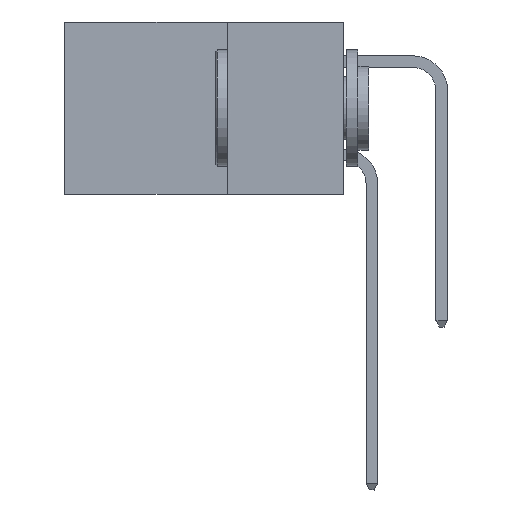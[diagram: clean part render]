
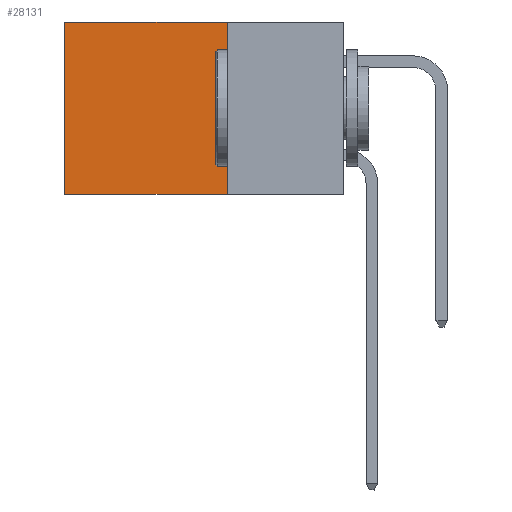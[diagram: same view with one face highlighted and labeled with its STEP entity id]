
A CAD part, left-side view. The second image highlights one B-rep face of the part: STEP entity #28131.
In plain terms, the highlighted planar face has unit normal (-1, 0, 0).
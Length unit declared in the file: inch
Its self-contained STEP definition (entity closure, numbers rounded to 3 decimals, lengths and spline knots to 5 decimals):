
#2382 = VECTOR ( 'NONE', #5284, 39.37008 ) ;
#3113 = CARTESIAN_POINT ( 'NONE',  ( 0.298, 0.6, 0. ) ) ;
#5284 = DIRECTION ( 'NONE',  ( 0., 0., -1. ) ) ;
#5970 = DIRECTION ( 'NONE',  ( 1., 0., 0. ) ) ;
#7076 = LINE ( 'NONE', #7590, #25088 ) ;
#7232 = CARTESIAN_POINT ( 'NONE',  ( 0.298, 0.25, -0.37 ) ) ;
#7590 = CARTESIAN_POINT ( 'NONE',  ( 0.298, 0.6, 0. ) ) ;
#7758 = VERTEX_POINT ( 'NONE', #3113 ) ;
#7760 = CARTESIAN_POINT ( 'NONE',  ( 0.298, 0.25, 0. ) ) ;
#7914 = ORIENTED_EDGE ( 'NONE', *, *, #15413, .T. ) ;
#8368 = EDGE_CURVE ( 'NONE', #19452, #11345, #15502, .T. ) ;
#10420 = CARTESIAN_POINT ( 'NONE',  ( 0.298, 0.6, -0.37 ) ) ;
#10487 = CARTESIAN_POINT ( 'NONE',  ( 0.298, 0.25, 0. ) ) ;
#10647 = FACE_OUTER_BOUND ( 'NONE', #14388, .T. ) ;
#11345 = VERTEX_POINT ( 'NONE', #16729 ) ;
#11483 = LINE ( 'NONE', #7232, #30175 ) ;
#12936 = DIRECTION ( 'NONE',  ( 0., 1., 0. ) ) ;
#13185 = ORIENTED_EDGE ( 'NONE', *, *, #17629, .F. ) ;
#13263 = PLANE ( 'NONE',  #22134 ) ;
#14388 = EDGE_LOOP ( 'NONE', ( #24601, #13185, #17001, #7914 ) ) ;
#14979 = DIRECTION ( 'NONE',  ( 0., 0., -1. ) ) ;
#15413 = EDGE_CURVE ( 'NONE', #19452, #7758, #17000, .T. ) ;
#15502 = LINE ( 'NONE', #7760, #2382 ) ;
#16729 = CARTESIAN_POINT ( 'NONE',  ( 0.298, 0.25, -0.37 ) ) ;
#17000 = LINE ( 'NONE', #10487, #22762 ) ;
#17001 = ORIENTED_EDGE ( 'NONE', *, *, #8368, .F. ) ;
#17629 = EDGE_CURVE ( 'NONE', #11345, #27325, #11483, .T. ) ;
#19452 = VERTEX_POINT ( 'NONE', #31330 ) ;
#20705 = CARTESIAN_POINT ( 'NONE',  ( 0.298, 0.25, 0. ) ) ;
#21943 = DIRECTION ( 'NONE',  ( 0., 1., 0. ) ) ;
#22134 = AXIS2_PLACEMENT_3D ( 'NONE', #20705, #5970, #23171 ) ;
#22762 = VECTOR ( 'NONE', #12936, 39.37008 ) ;
#22870 = EDGE_CURVE ( 'NONE', #7758, #27325, #7076, .T. ) ;
#23171 = DIRECTION ( 'NONE',  ( 0., 0., -1. ) ) ;
#24601 = ORIENTED_EDGE ( 'NONE', *, *, #22870, .T. ) ;
#25088 = VECTOR ( 'NONE', #14979, 39.37008 ) ;
#27325 = VERTEX_POINT ( 'NONE', #10420 ) ;
#28131 = ADVANCED_FACE ( 'NONE', ( #10647 ), #13263, .F. ) ;
#30175 = VECTOR ( 'NONE', #21943, 39.37008 ) ;
#31330 = CARTESIAN_POINT ( 'NONE',  ( 0.298, 0.25, 0. ) ) ;
